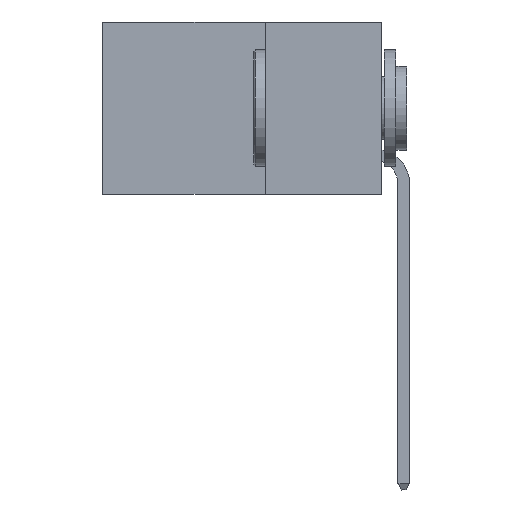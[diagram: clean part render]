
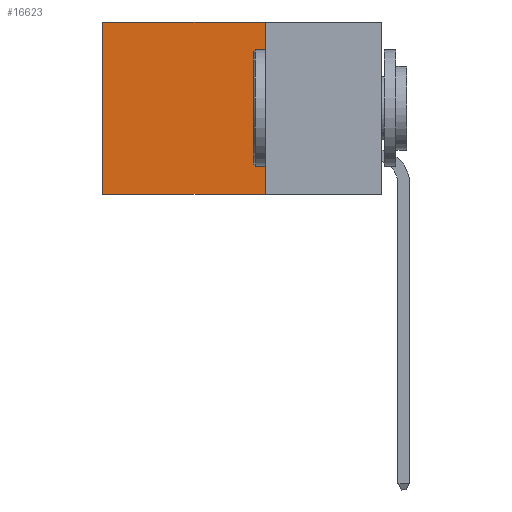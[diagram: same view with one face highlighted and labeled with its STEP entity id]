
A CAD part, left-side view. The second image highlights one B-rep face of the part: STEP entity #16623.
In plain terms, the highlighted planar face has unit normal (-1, 0, 0).
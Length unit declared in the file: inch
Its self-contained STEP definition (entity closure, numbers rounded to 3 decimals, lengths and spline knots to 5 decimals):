
#604 = VECTOR ( 'NONE', #15858, 39.37008 ) ;
#1084 = DIRECTION ( 'NONE',  ( 1., 0., 0. ) ) ;
#1287 = VERTEX_POINT ( 'NONE', #17307 ) ;
#1993 = CARTESIAN_POINT ( 'NONE',  ( 0.2875, 0.25, -0.37 ) ) ;
#2074 = LINE ( 'NONE', #21591, #6643 ) ;
#3545 = EDGE_CURVE ( 'NONE', #1287, #20877, #7421, .T. ) ;
#3637 = ORIENTED_EDGE ( 'NONE', *, *, #9939, .T. ) ;
#3944 = DIRECTION ( 'NONE',  ( 0., 1., 0. ) ) ;
#4266 = CARTESIAN_POINT ( 'NONE',  ( 0.2875, 0.6, 0. ) ) ;
#4934 = CARTESIAN_POINT ( 'NONE',  ( 0.2875, 0.6, -0.37 ) ) ;
#5344 = ORIENTED_EDGE ( 'NONE', *, *, #3545, .T. ) ;
#6318 = ORIENTED_EDGE ( 'NONE', *, *, #24604, .F. ) ;
#6643 = VECTOR ( 'NONE', #8203, 39.37008 ) ;
#7004 = PLANE ( 'NONE',  #17552 ) ;
#7421 = LINE ( 'NONE', #4266, #604 ) ;
#7436 = ORIENTED_EDGE ( 'NONE', *, *, #18179, .F. ) ;
#8203 = DIRECTION ( 'NONE',  ( 0., 0., -1. ) ) ;
#9939 = EDGE_CURVE ( 'NONE', #24768, #1287, #14233, .T. ) ;
#10321 = EDGE_LOOP ( 'NONE', ( #5344, #7436, #6318, #3637 ) ) ;
#10634 = CARTESIAN_POINT ( 'NONE',  ( 0.2875, 0.25, 0. ) ) ;
#10915 = DIRECTION ( 'NONE',  ( 0., 0., -1. ) ) ;
#10921 = VECTOR ( 'NONE', #3944, 39.37008 ) ;
#11094 = DIRECTION ( 'NONE',  ( 0., 1., 0. ) ) ;
#14233 = LINE ( 'NONE', #22485, #20534 ) ;
#14676 = CARTESIAN_POINT ( 'NONE',  ( 0.2875, 0.25, 0. ) ) ;
#15408 = LINE ( 'NONE', #17469, #10921 ) ;
#15858 = DIRECTION ( 'NONE',  ( 0., 0., -1. ) ) ;
#16249 = VERTEX_POINT ( 'NONE', #1993 ) ;
#16623 = ADVANCED_FACE ( 'NONE', ( #23896 ), #7004, .F. ) ;
#17307 = CARTESIAN_POINT ( 'NONE',  ( 0.2875, 0.6, 0. ) ) ;
#17469 = CARTESIAN_POINT ( 'NONE',  ( 0.2875, 0.25, -0.37 ) ) ;
#17552 = AXIS2_PLACEMENT_3D ( 'NONE', #14676, #1084, #10915 ) ;
#18179 = EDGE_CURVE ( 'NONE', #16249, #20877, #15408, .T. ) ;
#20534 = VECTOR ( 'NONE', #11094, 39.37008 ) ;
#20877 = VERTEX_POINT ( 'NONE', #4934 ) ;
#21591 = CARTESIAN_POINT ( 'NONE',  ( 0.2875, 0.25, 0. ) ) ;
#22485 = CARTESIAN_POINT ( 'NONE',  ( 0.2875, 0.25, 0. ) ) ;
#23896 = FACE_OUTER_BOUND ( 'NONE', #10321, .T. ) ;
#24604 = EDGE_CURVE ( 'NONE', #24768, #16249, #2074, .T. ) ;
#24768 = VERTEX_POINT ( 'NONE', #10634 ) ;
